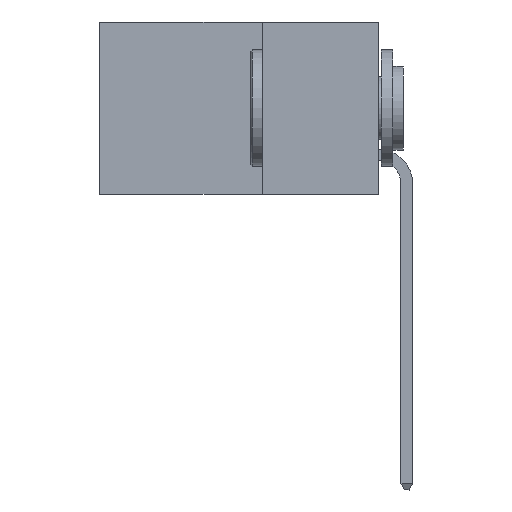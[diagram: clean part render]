
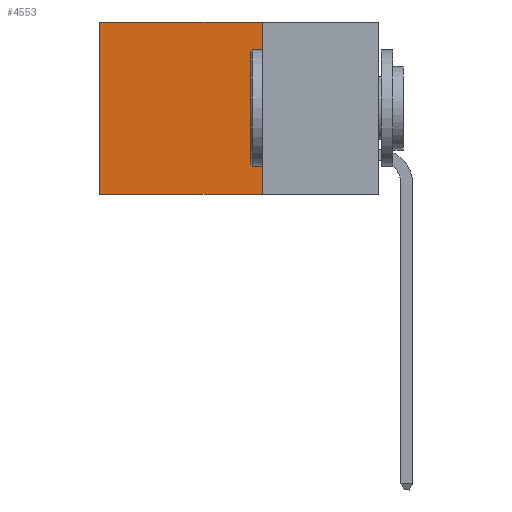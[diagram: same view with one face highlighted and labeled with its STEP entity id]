
A CAD part, left-side view. The second image highlights one B-rep face of the part: STEP entity #4553.
In plain terms, the highlighted planar face has unit normal (-1, 0, 0).
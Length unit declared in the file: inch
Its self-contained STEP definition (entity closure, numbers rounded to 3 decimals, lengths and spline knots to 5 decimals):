
#258 = AXIS2_PLACEMENT_3D ( 'NONE', #2391, #10682, #503 ) ;
#503 = DIRECTION ( 'NONE',  ( 0., 0., -1. ) ) ;
#847 = VECTOR ( 'NONE', #6671, 39.37008 ) ;
#1192 = VERTEX_POINT ( 'NONE', #10228 ) ;
#1799 = LINE ( 'NONE', #7269, #4715 ) ;
#2391 = CARTESIAN_POINT ( 'NONE',  ( 0.2615, 0.25, -0.37 ) ) ;
#2663 = DIRECTION ( 'NONE',  ( 0., 1., 0. ) ) ;
#2783 = LINE ( 'NONE', #4432, #4148 ) ;
#3444 = CARTESIAN_POINT ( 'NONE',  ( 0.2615, 0.25, -0.37 ) ) ;
#3771 = CARTESIAN_POINT ( 'NONE',  ( 0.2615, 0.6, -0.37 ) ) ;
#4104 = EDGE_LOOP ( 'NONE', ( #10363, #8359, #6730, #6362 ) ) ;
#4148 = VECTOR ( 'NONE', #9183, 39.37008 ) ;
#4418 = CARTESIAN_POINT ( 'NONE',  ( 0.2615, 0.6, 0. ) ) ;
#4432 = CARTESIAN_POINT ( 'NONE',  ( 0.2615, 0.25, 0. ) ) ;
#4553 = ADVANCED_FACE ( 'NONE', ( #10747 ), #9762, .F. ) ;
#4698 = LINE ( 'NONE', #3771, #847 ) ;
#4715 = VECTOR ( 'NONE', #2663, 39.37008 ) ;
#5079 = EDGE_CURVE ( 'NONE', #5535, #5281, #7983, .T. ) ;
#5281 = VERTEX_POINT ( 'NONE', #6860 ) ;
#5535 = VERTEX_POINT ( 'NONE', #7157 ) ;
#6225 = DIRECTION ( 'NONE',  ( 0., 0., -1. ) ) ;
#6362 = ORIENTED_EDGE ( 'NONE', *, *, #7937, .T. ) ;
#6671 = DIRECTION ( 'NONE',  ( 0., 0., -1. ) ) ;
#6730 = ORIENTED_EDGE ( 'NONE', *, *, #5079, .F. ) ;
#6860 = CARTESIAN_POINT ( 'NONE',  ( 0.2615, 0.25, -0.37 ) ) ;
#7076 = VERTEX_POINT ( 'NONE', #4418 ) ;
#7157 = CARTESIAN_POINT ( 'NONE',  ( 0.2615, 0.25, 0. ) ) ;
#7174 = EDGE_CURVE ( 'NONE', #5281, #1192, #1799, .T. ) ;
#7269 = CARTESIAN_POINT ( 'NONE',  ( 0.2615, 0.25, -0.37 ) ) ;
#7275 = EDGE_CURVE ( 'NONE', #7076, #1192, #4698, .T. ) ;
#7937 = EDGE_CURVE ( 'NONE', #5535, #7076, #2783, .T. ) ;
#7983 = LINE ( 'NONE', #3444, #10914 ) ;
#8359 = ORIENTED_EDGE ( 'NONE', *, *, #7174, .F. ) ;
#9183 = DIRECTION ( 'NONE',  ( 0., 1., 0. ) ) ;
#9762 = PLANE ( 'NONE',  #258 ) ;
#10228 = CARTESIAN_POINT ( 'NONE',  ( 0.2615, 0.6, -0.37 ) ) ;
#10363 = ORIENTED_EDGE ( 'NONE', *, *, #7275, .T. ) ;
#10682 = DIRECTION ( 'NONE',  ( 1., 0., 0. ) ) ;
#10747 = FACE_OUTER_BOUND ( 'NONE', #4104, .T. ) ;
#10914 = VECTOR ( 'NONE', #6225, 39.37008 ) ;
